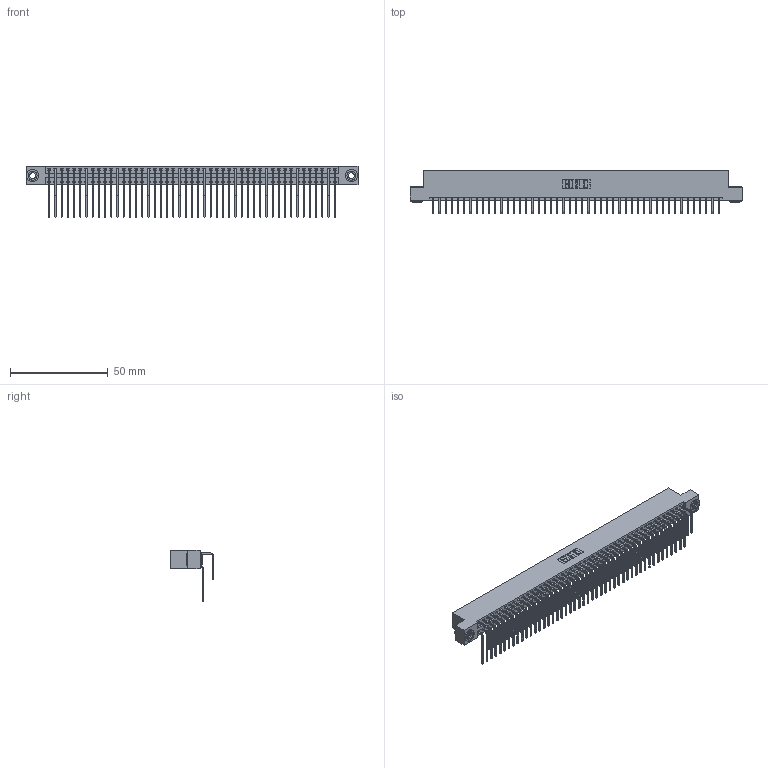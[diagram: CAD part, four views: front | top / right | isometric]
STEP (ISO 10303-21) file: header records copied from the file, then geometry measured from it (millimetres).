
FILE_DESCRIPTION (( 'STEP AP203' ), '1' );
FILE_NAME ('396-094-558-203.STEP', '2019-11-03T14:52:31', ( '' ), ( '' ), 'SwSTEP 2.0', 'SolidWorks 2016', '' );
FILE_SCHEMA (( 'CONFIG_CONTROL_DESIGN' ));
Length unit declared in the file: inch
Products named in the file (5): 346 Part_Flush Mounting Lugs - 0.156 Dia-TH; 345-292-001_558 559 Tail - 1; 345-292-001_558 Tail - 2; 396-094-558-203; 345-250-002_345-250-002-102
Assembly tree (97 placements, depth 2):
  396-094-558-203
    346 Part_Flush Mounting Lugs - 0.156 Dia-TH
    345-292-001_558 559 Tail - 1  x47
    345-292-001_558 Tail - 2  x47
    345-250-002_345-250-002-102  x2
Bounding box: 169.8 x 22.16 x 26.16 mm (x, y, z)
Volume: 17158 mm3; surface area: 26479 mm2
Topology: 97 solids, 97 shells, 5236 faces, 15539 edges, 10230 vertices
Faces by surface type: plane 3564, cylinder 1664, cone 8
Entity records: 32434 total; most frequent: CARTESIAN_POINT 5366, ORIENTED_EDGE 5242, DIRECTION 4783, EDGE_CURVE 2621, VECTOR 2237, LINE 2237, VERTEX_POINT 1742, AXIS2_PLACEMENT_3D 1273
